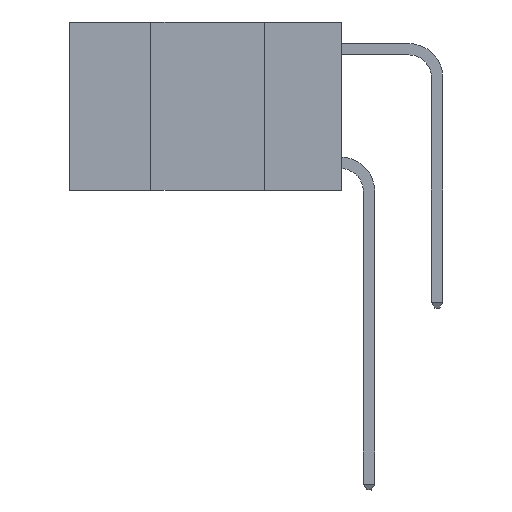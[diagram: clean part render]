
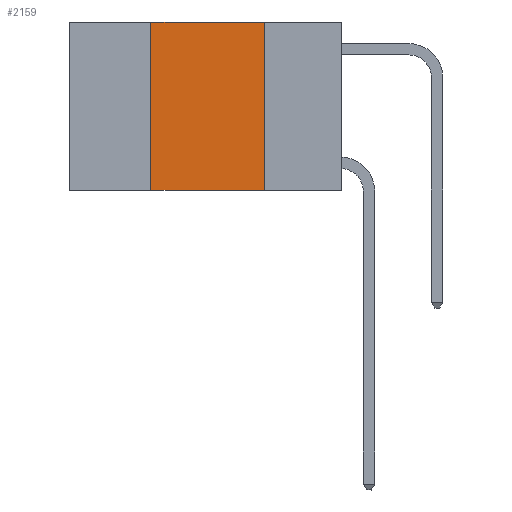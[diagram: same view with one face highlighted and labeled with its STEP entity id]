
A CAD part, left-side view. The second image highlights one B-rep face of the part: STEP entity #2159.
In plain terms, the highlighted planar face has unit normal (-1, 0, 0).
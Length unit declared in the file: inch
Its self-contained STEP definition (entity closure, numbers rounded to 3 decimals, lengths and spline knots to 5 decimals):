
#125 = PLANE ( 'NONE',  #16153 ) ;
#419 = DIRECTION ( 'NONE',  ( 0., -1., 0. ) ) ;
#1622 = LINE ( 'NONE', #14567, #14793 ) ;
#2159 = ADVANCED_FACE ( 'NONE', ( #11802 ), #125, .F. ) ;
#2198 = VECTOR ( 'NONE', #14757, 39.37008 ) ;
#3516 = LINE ( 'NONE', #5491, #12491 ) ;
#4844 = VECTOR ( 'NONE', #419, 39.37008 ) ;
#5385 = DIRECTION ( 'NONE',  ( 0., 0., -1. ) ) ;
#5491 = CARTESIAN_POINT ( 'NONE',  ( 0., 0.42, 0. ) ) ;
#5664 = LINE ( 'NONE', #7131, #2198 ) ;
#5957 = EDGE_CURVE ( 'NONE', #13883, #8278, #5664, .T. ) ;
#6497 = EDGE_CURVE ( 'NONE', #12164, #13883, #7831, .T. ) ;
#6582 = CARTESIAN_POINT ( 'NONE',  ( 0., 0.42, -0.37 ) ) ;
#6771 = DIRECTION ( 'NONE',  ( 0., 0., 1. ) ) ;
#7131 = CARTESIAN_POINT ( 'NONE',  ( 0., 0.17, 0. ) ) ;
#7831 = LINE ( 'NONE', #9441, #4844 ) ;
#8278 = VERTEX_POINT ( 'NONE', #12863 ) ;
#9142 = ORIENTED_EDGE ( 'NONE', *, *, #6497, .F. ) ;
#9160 = CARTESIAN_POINT ( 'NONE',  ( 0., 0.6, 0. ) ) ;
#9441 = CARTESIAN_POINT ( 'NONE',  ( 0., 0.6, 0. ) ) ;
#9544 = ORIENTED_EDGE ( 'NONE', *, *, #13337, .T. ) ;
#9737 = EDGE_CURVE ( 'NONE', #14133, #12164, #3516, .T. ) ;
#9796 = CARTESIAN_POINT ( 'NONE',  ( 0., 0.42, 0. ) ) ;
#11802 = FACE_OUTER_BOUND ( 'NONE', #15013, .T. ) ;
#12119 = ORIENTED_EDGE ( 'NONE', *, *, #5957, .F. ) ;
#12164 = VERTEX_POINT ( 'NONE', #9796 ) ;
#12410 = CARTESIAN_POINT ( 'NONE',  ( 0., 0.17, 0. ) ) ;
#12491 = VECTOR ( 'NONE', #6771, 39.37008 ) ;
#12863 = CARTESIAN_POINT ( 'NONE',  ( 0., 0.17, -0.37 ) ) ;
#13010 = DIRECTION ( 'NONE',  ( 1., 0., 0. ) ) ;
#13337 = EDGE_CURVE ( 'NONE', #14133, #8278, #1622, .T. ) ;
#13883 = VERTEX_POINT ( 'NONE', #12410 ) ;
#14133 = VERTEX_POINT ( 'NONE', #6582 ) ;
#14567 = CARTESIAN_POINT ( 'NONE',  ( 0., 0.6, -0.37 ) ) ;
#14757 = DIRECTION ( 'NONE',  ( 0., 0., -1. ) ) ;
#14793 = VECTOR ( 'NONE', #15841, 39.37008 ) ;
#15013 = EDGE_LOOP ( 'NONE', ( #12119, #9142, #15869, #9544 ) ) ;
#15841 = DIRECTION ( 'NONE',  ( 0., -1., 0. ) ) ;
#15869 = ORIENTED_EDGE ( 'NONE', *, *, #9737, .F. ) ;
#16153 = AXIS2_PLACEMENT_3D ( 'NONE', #9160, #13010, #5385 ) ;
